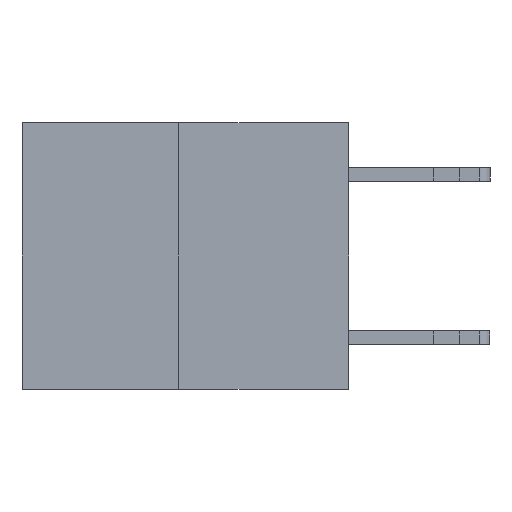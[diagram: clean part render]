
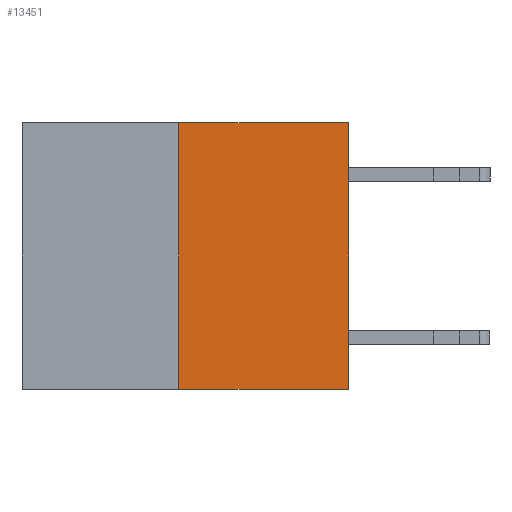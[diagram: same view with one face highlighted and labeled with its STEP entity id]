
A CAD part, left-side view. The second image highlights one B-rep face of the part: STEP entity #13451.
In plain terms, the highlighted planar face has unit normal (-1, 0, 0).
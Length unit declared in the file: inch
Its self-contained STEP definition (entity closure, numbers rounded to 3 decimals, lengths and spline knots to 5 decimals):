
#157 = VERTEX_POINT ( 'NONE', #5966 ) ;
#171 = LINE ( 'NONE', #792, #6722 ) ;
#236 = DIRECTION ( 'NONE',  ( 0., 0., 1. ) ) ;
#290 = CARTESIAN_POINT ( 'NONE',  ( 0., 0., 0. ) ) ;
#626 = CARTESIAN_POINT ( 'NONE',  ( 0., 0.312, 0. ) ) ;
#792 = CARTESIAN_POINT ( 'NONE',  ( 0., 0.6, -0.49 ) ) ;
#939 = VECTOR ( 'NONE', #11841, 39.37008 ) ;
#2837 = ORIENTED_EDGE ( 'NONE', *, *, #15084, .F. ) ;
#3046 = DIRECTION ( 'NONE',  ( 0., 0., 1. ) ) ;
#3096 = VECTOR ( 'NONE', #236, 39.37008 ) ;
#4185 = CARTESIAN_POINT ( 'NONE',  ( 0., 0., 0. ) ) ;
#4311 = CARTESIAN_POINT ( 'NONE',  ( 0., 0.6, 0. ) ) ;
#5192 = ORIENTED_EDGE ( 'NONE', *, *, #14152, .T. ) ;
#5590 = CARTESIAN_POINT ( 'NONE',  ( 0., 0.6, 0. ) ) ;
#5868 = ORIENTED_EDGE ( 'NONE', *, *, #8552, .T. ) ;
#5956 = LINE ( 'NONE', #5590, #939 ) ;
#5966 = CARTESIAN_POINT ( 'NONE',  ( 0., 0., -0.49 ) ) ;
#5984 = FACE_OUTER_BOUND ( 'NONE', #6729, .T. ) ;
#6722 = VECTOR ( 'NONE', #12929, 39.37008 ) ;
#6729 = EDGE_LOOP ( 'NONE', ( #2837, #5868, #5192, #8207 ) ) ;
#7682 = VECTOR ( 'NONE', #3046, 39.37008 ) ;
#8000 = DIRECTION ( 'NONE',  ( 0., 0., -1. ) ) ;
#8110 = CARTESIAN_POINT ( 'NONE',  ( 0., 0.312, -0.49 ) ) ;
#8207 = ORIENTED_EDGE ( 'NONE', *, *, #8511, .F. ) ;
#8285 = LINE ( 'NONE', #290, #3096 ) ;
#8434 = VERTEX_POINT ( 'NONE', #626 ) ;
#8511 = EDGE_CURVE ( 'NONE', #8434, #9311, #5956, .T. ) ;
#8552 = EDGE_CURVE ( 'NONE', #11396, #157, #171, .T. ) ;
#9311 = VERTEX_POINT ( 'NONE', #4185 ) ;
#9983 = LINE ( 'NONE', #14984, #7682 ) ;
#10401 = PLANE ( 'NONE',  #11315 ) ;
#11315 = AXIS2_PLACEMENT_3D ( 'NONE', #4311, #15113, #8000 ) ;
#11396 = VERTEX_POINT ( 'NONE', #8110 ) ;
#11841 = DIRECTION ( 'NONE',  ( 0., -1., 0. ) ) ;
#12929 = DIRECTION ( 'NONE',  ( 0., -1., 0. ) ) ;
#13451 = ADVANCED_FACE ( 'NONE', ( #5984 ), #10401, .F. ) ;
#14152 = EDGE_CURVE ( 'NONE', #157, #9311, #8285, .T. ) ;
#14984 = CARTESIAN_POINT ( 'NONE',  ( 0., 0.312, -0.49 ) ) ;
#15084 = EDGE_CURVE ( 'NONE', #11396, #8434, #9983, .T. ) ;
#15113 = DIRECTION ( 'NONE',  ( 1., 0., 0. ) ) ;
